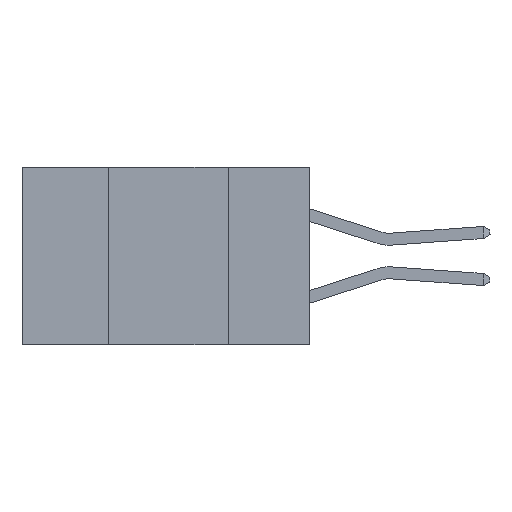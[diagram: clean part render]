
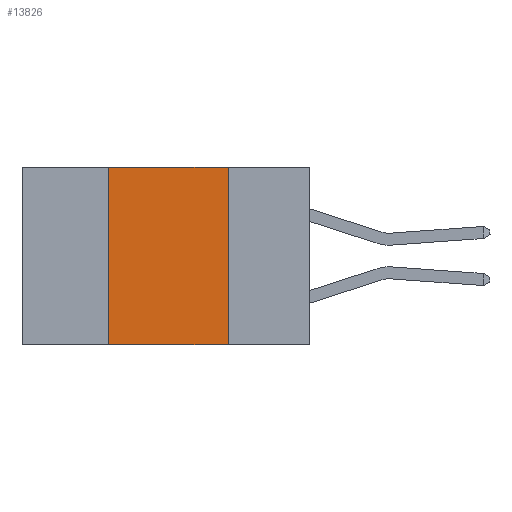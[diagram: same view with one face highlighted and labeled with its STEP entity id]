
A CAD part, left-side view. The second image highlights one B-rep face of the part: STEP entity #13826.
In plain terms, the highlighted planar face has unit normal (-1, 0, 0).
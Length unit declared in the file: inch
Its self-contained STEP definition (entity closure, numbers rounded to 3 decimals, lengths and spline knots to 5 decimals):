
#96 = VECTOR ( 'NONE', #569, 39.37008 ) ;
#569 = DIRECTION ( 'NONE',  ( 0., -1., 0. ) ) ;
#651 = CARTESIAN_POINT ( 'NONE',  ( 0., 0.6, -0.37 ) ) ;
#1802 = VERTEX_POINT ( 'NONE', #13777 ) ;
#2061 = CARTESIAN_POINT ( 'NONE',  ( 0., 0.17, -0.37 ) ) ;
#2354 = DIRECTION ( 'NONE',  ( 0., 0., -1. ) ) ;
#3278 = LINE ( 'NONE', #651, #96 ) ;
#3288 = EDGE_LOOP ( 'NONE', ( #5436, #3718, #8348, #12331 ) ) ;
#3718 = ORIENTED_EDGE ( 'NONE', *, *, #13986, .F. ) ;
#3730 = CARTESIAN_POINT ( 'NONE',  ( 0., 0.17, -0.37 ) ) ;
#5187 = VECTOR ( 'NONE', #13836, 39.37008 ) ;
#5320 = VECTOR ( 'NONE', #5924, 39.37008 ) ;
#5436 = ORIENTED_EDGE ( 'NONE', *, *, #14646, .F. ) ;
#5529 = CARTESIAN_POINT ( 'NONE',  ( 0., 0.42, 0. ) ) ;
#5924 = DIRECTION ( 'NONE',  ( 0., -1., 0. ) ) ;
#6337 = CARTESIAN_POINT ( 'NONE',  ( 0., 0.42, -0.37 ) ) ;
#6679 = CARTESIAN_POINT ( 'NONE',  ( 0., 0.6, 0. ) ) ;
#6938 = VERTEX_POINT ( 'NONE', #5529 ) ;
#7513 = LINE ( 'NONE', #2061, #13215 ) ;
#7915 = FACE_OUTER_BOUND ( 'NONE', #3288, .T. ) ;
#8348 = ORIENTED_EDGE ( 'NONE', *, *, #12533, .F. ) ;
#9018 = AXIS2_PLACEMENT_3D ( 'NONE', #9451, #9412, #9409 ) ;
#9409 = DIRECTION ( 'NONE',  ( 0., 0., -1. ) ) ;
#9412 = DIRECTION ( 'NONE',  ( 1., 0., 0. ) ) ;
#9451 = CARTESIAN_POINT ( 'NONE',  ( 0., 0.6, 0. ) ) ;
#9452 = PLANE ( 'NONE',  #9018 ) ;
#9483 = VERTEX_POINT ( 'NONE', #6337 ) ;
#11719 = LINE ( 'NONE', #13319, #5187 ) ;
#11781 = EDGE_CURVE ( 'NONE', #9483, #13182, #3278, .T. ) ;
#12331 = ORIENTED_EDGE ( 'NONE', *, *, #11781, .T. ) ;
#12533 = EDGE_CURVE ( 'NONE', #9483, #6938, #11719, .T. ) ;
#13182 = VERTEX_POINT ( 'NONE', #3730 ) ;
#13215 = VECTOR ( 'NONE', #2354, 39.37008 ) ;
#13319 = CARTESIAN_POINT ( 'NONE',  ( 0., 0.42, -0.37 ) ) ;
#13777 = CARTESIAN_POINT ( 'NONE',  ( 0., 0.17, 0. ) ) ;
#13826 = ADVANCED_FACE ( 'NONE', ( #7915 ), #9452, .F. ) ;
#13836 = DIRECTION ( 'NONE',  ( 0., 0., 1. ) ) ;
#13986 = EDGE_CURVE ( 'NONE', #6938, #1802, #14376, .T. ) ;
#14376 = LINE ( 'NONE', #6679, #5320 ) ;
#14646 = EDGE_CURVE ( 'NONE', #1802, #13182, #7513, .T. ) ;
